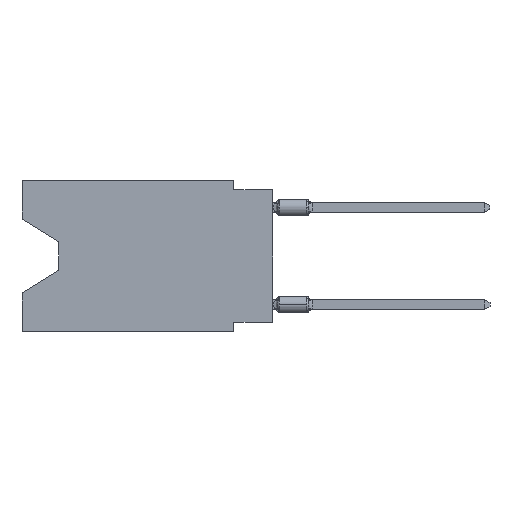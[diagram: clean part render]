
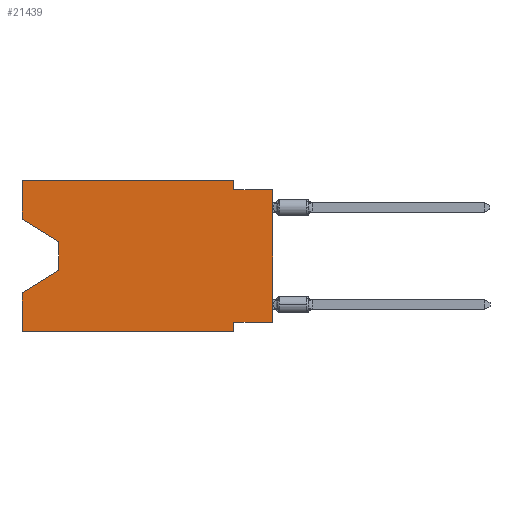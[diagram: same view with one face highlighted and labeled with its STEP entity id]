
A CAD part, left-side view. The second image highlights one B-rep face of the part: STEP entity #21439.
In plain terms, the highlighted planar face has unit normal (-1, 0, 0).
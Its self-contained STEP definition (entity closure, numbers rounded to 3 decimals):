
#143 = ORIENTED_EDGE ( 'NONE', *, *, #1137, .F. ) ;
#523 = LINE ( 'NONE', #2334, #24793 ) ;
#769 = ORIENTED_EDGE ( 'NONE', *, *, #23746, .F. ) ;
#1052 = VECTOR ( 'NONE', #6850, 1000. ) ;
#1137 = EDGE_CURVE ( 'NONE', #16066, #24531, #24628, .T. ) ;
#1463 = DIRECTION ( 'NONE',  ( 0., 0., 1. ) ) ;
#1705 = CARTESIAN_POINT ( 'NONE',  ( 0., 16.383, -7.36 ) ) ;
#1765 = DIRECTION ( 'NONE',  ( 0., -1., 0. ) ) ;
#1886 = EDGE_CURVE ( 'NONE', #2404, #6709, #6227, .T. ) ;
#2194 = CARTESIAN_POINT ( 'NONE',  ( 0., 2.54, 0. ) ) ;
#2334 = CARTESIAN_POINT ( 'NONE',  ( 0., 13.97, -4.013 ) ) ;
#2404 = VERTEX_POINT ( 'NONE', #16860 ) ;
#3670 = VECTOR ( 'NONE', #13322, 1000. ) ;
#3732 = VERTEX_POINT ( 'NONE', #8151 ) ;
#4174 = VECTOR ( 'NONE', #17052, 1000. ) ;
#4333 = DIRECTION ( 'NONE',  ( 1., 0., 0. ) ) ;
#4463 = CARTESIAN_POINT ( 'NONE',  ( 0., 16.383, 0. ) ) ;
#4808 = VECTOR ( 'NONE', #21806, 1000. ) ;
#4926 = EDGE_CURVE ( 'NONE', #15035, #20356, #12032, .T. ) ;
#5065 = CARTESIAN_POINT ( 'NONE',  ( 0., 2.54, -9.906 ) ) ;
#5358 = VECTOR ( 'NONE', #14589, 1000. ) ;
#5590 = CARTESIAN_POINT ( 'NONE',  ( 0., 16.383, -2.546 ) ) ;
#5591 = DIRECTION ( 'NONE',  ( 0., 0., 1. ) ) ;
#5631 = ORIENTED_EDGE ( 'NONE', *, *, #20297, .F. ) ;
#5757 = DIRECTION ( 'NONE',  ( 0., 0., -1. ) ) ;
#5772 = DIRECTION ( 'NONE',  ( 0., -1., 0. ) ) ;
#6183 = VECTOR ( 'NONE', #5772, 1000. ) ;
#6227 = LINE ( 'NONE', #12195, #15563 ) ;
#6266 = PLANE ( 'NONE',  #14305 ) ;
#6501 = CARTESIAN_POINT ( 'NONE',  ( 0., 16.383, -9.906 ) ) ;
#6709 = VERTEX_POINT ( 'NONE', #5065 ) ;
#6742 = VERTEX_POINT ( 'NONE', #6501 ) ;
#6850 = DIRECTION ( 'NONE',  ( 0., 0., -1. ) ) ;
#6925 = EDGE_CURVE ( 'NONE', #21540, #21923, #13381, .T. ) ;
#7673 = DIRECTION ( 'NONE',  ( 0., -0.855, -0.519 ) ) ;
#7674 = CARTESIAN_POINT ( 'NONE',  ( 0., 16.383, 0. ) ) ;
#7803 = VECTOR ( 'NONE', #7673, 1000. ) ;
#7810 = LINE ( 'NONE', #5590, #7803 ) ;
#8151 = CARTESIAN_POINT ( 'NONE',  ( 0., 13.97, -5.893 ) ) ;
#8214 = CARTESIAN_POINT ( 'NONE',  ( 0., 2.54, -0.635 ) ) ;
#8577 = CARTESIAN_POINT ( 'NONE',  ( 0., 16.383, 0. ) ) ;
#8895 = LINE ( 'NONE', #14716, #5358 ) ;
#10175 = VECTOR ( 'NONE', #1765, 1000. ) ;
#11548 = CARTESIAN_POINT ( 'NONE',  ( 0., 0., 0. ) ) ;
#11598 = LINE ( 'NONE', #19508, #10175 ) ;
#11743 = ORIENTED_EDGE ( 'NONE', *, *, #1886, .F. ) ;
#12032 = LINE ( 'NONE', #7674, #14660 ) ;
#12059 = CARTESIAN_POINT ( 'NONE',  ( 0., 0., -0.635 ) ) ;
#12195 = CARTESIAN_POINT ( 'NONE',  ( 0., 2.54, -9.906 ) ) ;
#13322 = DIRECTION ( 'NONE',  ( 0., 0., 1. ) ) ;
#13381 = LINE ( 'NONE', #11548, #14230 ) ;
#13735 = ORIENTED_EDGE ( 'NONE', *, *, #25212, .T. ) ;
#14230 = VECTOR ( 'NONE', #1463, 1000. ) ;
#14305 = AXIS2_PLACEMENT_3D ( 'NONE', #23550, #4333, #5757 ) ;
#14589 = DIRECTION ( 'NONE',  ( 0., 1., 0. ) ) ;
#14659 = EDGE_LOOP ( 'NONE', ( #18777, #13735, #19542, #769, #16269, #11743, #24870, #16064, #5631, #143, #24730, #15079 ) ) ;
#14660 = VECTOR ( 'NONE', #5591, 1000. ) ;
#14716 = CARTESIAN_POINT ( 'NONE',  ( 0., 0., -9.271 ) ) ;
#15035 = VERTEX_POINT ( 'NONE', #24736 ) ;
#15079 = ORIENTED_EDGE ( 'NONE', *, *, #4926, .F. ) ;
#15136 = LINE ( 'NONE', #23566, #6183 ) ;
#15229 = EDGE_CURVE ( 'NONE', #20356, #16066, #15136, .T. ) ;
#15563 = VECTOR ( 'NONE', #18047, 1000. ) ;
#16053 = DIRECTION ( 'NONE',  ( 0., 0., -1. ) ) ;
#16064 = ORIENTED_EDGE ( 'NONE', *, *, #6925, .T. ) ;
#16066 = VERTEX_POINT ( 'NONE', #2194 ) ;
#16269 = ORIENTED_EDGE ( 'NONE', *, *, #21868, .T. ) ;
#16628 = EDGE_CURVE ( 'NONE', #3732, #17265, #22639, .T. ) ;
#16860 = CARTESIAN_POINT ( 'NONE',  ( 0., 2.54, -9.271 ) ) ;
#16973 = CARTESIAN_POINT ( 'NONE',  ( 0., 2.54, 0. ) ) ;
#17052 = DIRECTION ( 'NONE',  ( 0., 0.855, -0.519 ) ) ;
#17194 = VERTEX_POINT ( 'NONE', #21784 ) ;
#17265 = VERTEX_POINT ( 'NONE', #1705 ) ;
#18047 = DIRECTION ( 'NONE',  ( 0., 0., -1. ) ) ;
#18339 = CARTESIAN_POINT ( 'NONE',  ( 0., 0., -9.271 ) ) ;
#18494 = CARTESIAN_POINT ( 'NONE',  ( 0., 13.97, -5.893 ) ) ;
#18656 = EDGE_CURVE ( 'NONE', #21540, #2404, #8895, .T. ) ;
#18777 = ORIENTED_EDGE ( 'NONE', *, *, #24707, .T. ) ;
#19508 = CARTESIAN_POINT ( 'NONE',  ( 0., 0., -0.635 ) ) ;
#19542 = ORIENTED_EDGE ( 'NONE', *, *, #16628, .T. ) ;
#20297 = EDGE_CURVE ( 'NONE', #24531, #21923, #11598, .T. ) ;
#20356 = VERTEX_POINT ( 'NONE', #4463 ) ;
#21439 = ADVANCED_FACE ( 'NONE', ( #24049 ), #6266, .F. ) ;
#21540 = VERTEX_POINT ( 'NONE', #18339 ) ;
#21674 = CARTESIAN_POINT ( 'NONE',  ( 0., 16.383, -9.906 ) ) ;
#21784 = CARTESIAN_POINT ( 'NONE',  ( 0., 13.97, -4.013 ) ) ;
#21806 = DIRECTION ( 'NONE',  ( 0., -1., 0. ) ) ;
#21868 = EDGE_CURVE ( 'NONE', #6742, #6709, #25209, .T. ) ;
#21923 = VERTEX_POINT ( 'NONE', #12059 ) ;
#22639 = LINE ( 'NONE', #18494, #4174 ) ;
#23192 = LINE ( 'NONE', #8577, #3670 ) ;
#23550 = CARTESIAN_POINT ( 'NONE',  ( 0., 16.383, 0. ) ) ;
#23566 = CARTESIAN_POINT ( 'NONE',  ( 0., 16.383, 0. ) ) ;
#23746 = EDGE_CURVE ( 'NONE', #6742, #17265, #23192, .T. ) ;
#24049 = FACE_OUTER_BOUND ( 'NONE', #14659, .T. ) ;
#24531 = VERTEX_POINT ( 'NONE', #8214 ) ;
#24628 = LINE ( 'NONE', #16973, #1052 ) ;
#24707 = EDGE_CURVE ( 'NONE', #15035, #17194, #7810, .T. ) ;
#24730 = ORIENTED_EDGE ( 'NONE', *, *, #15229, .F. ) ;
#24736 = CARTESIAN_POINT ( 'NONE',  ( 0., 16.383, -2.546 ) ) ;
#24793 = VECTOR ( 'NONE', #16053, 1000. ) ;
#24870 = ORIENTED_EDGE ( 'NONE', *, *, #18656, .F. ) ;
#25209 = LINE ( 'NONE', #21674, #4808 ) ;
#25212 = EDGE_CURVE ( 'NONE', #17194, #3732, #523, .T. ) ;
